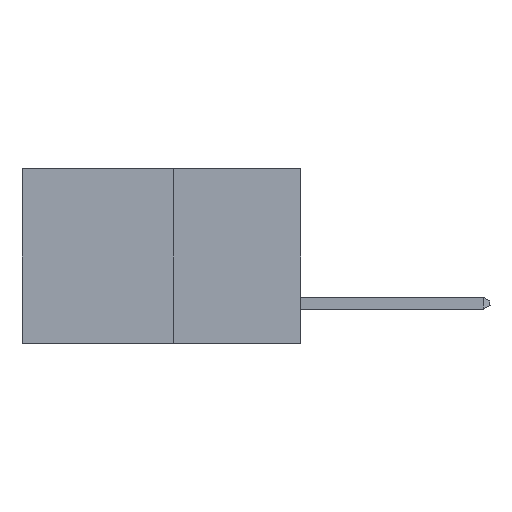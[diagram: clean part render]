
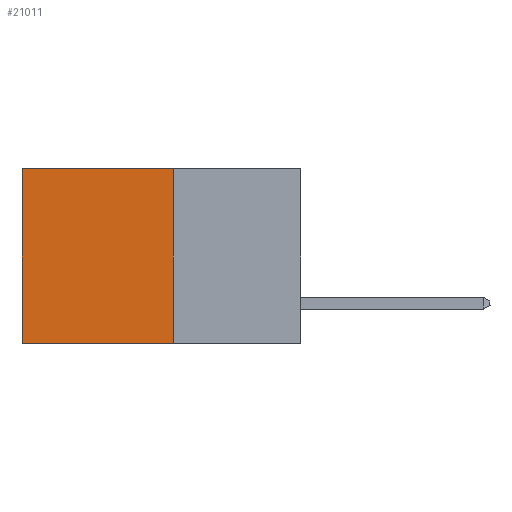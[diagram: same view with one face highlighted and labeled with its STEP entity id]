
A CAD part, left-side view. The second image highlights one B-rep face of the part: STEP entity #21011.
In plain terms, the highlighted planar face has unit normal (-1, 0, 0).
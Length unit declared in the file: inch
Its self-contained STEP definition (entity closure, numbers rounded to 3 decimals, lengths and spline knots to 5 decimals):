
#213 = VERTEX_POINT ( 'NONE', #2288 ) ;
#1019 = AXIS2_PLACEMENT_3D ( 'NONE', #17924, #7746, #19552 ) ;
#1645 = VECTOR ( 'NONE', #17551, 39.37008 ) ;
#2288 = CARTESIAN_POINT ( 'NONE',  ( 0.277, 0.59, 0. ) ) ;
#3568 = CARTESIAN_POINT ( 'NONE',  ( 0.277, 0.59, -0.37 ) ) ;
#5319 = DIRECTION ( 'NONE',  ( 0., 1., 0. ) ) ;
#5581 = ORIENTED_EDGE ( 'NONE', *, *, #19910, .T. ) ;
#7746 = DIRECTION ( 'NONE',  ( 1., 0., 0. ) ) ;
#7806 = VERTEX_POINT ( 'NONE', #8034 ) ;
#7931 = FACE_OUTER_BOUND ( 'NONE', #17787, .T. ) ;
#8034 = CARTESIAN_POINT ( 'NONE',  ( 0.277, 0.27, -0.37 ) ) ;
#8093 = LINE ( 'NONE', #15801, #8622 ) ;
#8622 = VECTOR ( 'NONE', #14017, 39.37008 ) ;
#9440 = VECTOR ( 'NONE', #14000, 39.37008 ) ;
#9629 = VECTOR ( 'NONE', #5319, 39.37008 ) ;
#10184 = LINE ( 'NONE', #17222, #9629 ) ;
#10735 = VERTEX_POINT ( 'NONE', #3568 ) ;
#11223 = EDGE_CURVE ( 'NONE', #20570, #213, #10184, .T. ) ;
#12808 = PLANE ( 'NONE',  #1019 ) ;
#13821 = ORIENTED_EDGE ( 'NONE', *, *, #20208, .F. ) ;
#13959 = LINE ( 'NONE', #20623, #9440 ) ;
#14000 = DIRECTION ( 'NONE',  ( 0., 0., -1. ) ) ;
#14017 = DIRECTION ( 'NONE',  ( 0., 1., 0. ) ) ;
#14858 = EDGE_CURVE ( 'NONE', #20570, #7806, #15223, .T. ) ;
#14952 = CARTESIAN_POINT ( 'NONE',  ( 0.277, 0.27, 0. ) ) ;
#15223 = LINE ( 'NONE', #20730, #1645 ) ;
#15801 = CARTESIAN_POINT ( 'NONE',  ( 0.277, 0.27, -0.37 ) ) ;
#15958 = ORIENTED_EDGE ( 'NONE', *, *, #14858, .F. ) ;
#17036 = ORIENTED_EDGE ( 'NONE', *, *, #11223, .T. ) ;
#17222 = CARTESIAN_POINT ( 'NONE',  ( 0.277, 0.27, 0. ) ) ;
#17551 = DIRECTION ( 'NONE',  ( 0., 0., -1. ) ) ;
#17787 = EDGE_LOOP ( 'NONE', ( #5581, #13821, #15958, #17036 ) ) ;
#17924 = CARTESIAN_POINT ( 'NONE',  ( 0.277, 0.27, -0.37 ) ) ;
#19552 = DIRECTION ( 'NONE',  ( 0., 0., -1. ) ) ;
#19910 = EDGE_CURVE ( 'NONE', #213, #10735, #13959, .T. ) ;
#20208 = EDGE_CURVE ( 'NONE', #7806, #10735, #8093, .T. ) ;
#20570 = VERTEX_POINT ( 'NONE', #14952 ) ;
#20623 = CARTESIAN_POINT ( 'NONE',  ( 0.277, 0.59, -0.37 ) ) ;
#20730 = CARTESIAN_POINT ( 'NONE',  ( 0.277, 0.27, -0.37 ) ) ;
#21011 = ADVANCED_FACE ( 'NONE', ( #7931 ), #12808, .F. ) ;
